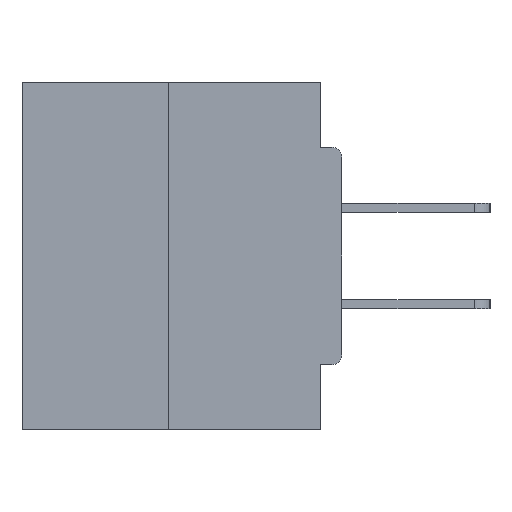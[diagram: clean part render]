
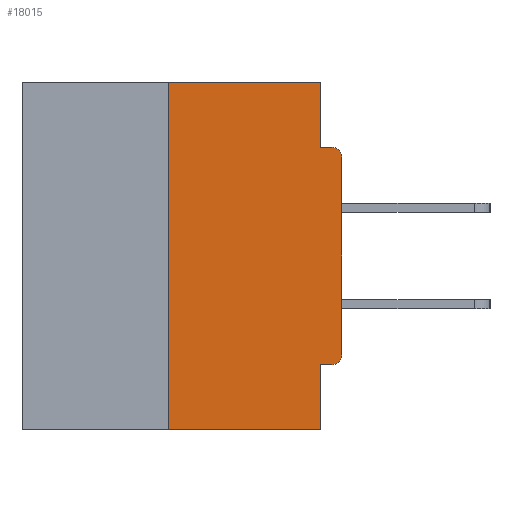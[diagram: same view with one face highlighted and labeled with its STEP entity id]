
A CAD part, left-side view. The second image highlights one B-rep face of the part: STEP entity #18015.
In plain terms, the highlighted planar face has unit normal (-1, 0, 0).
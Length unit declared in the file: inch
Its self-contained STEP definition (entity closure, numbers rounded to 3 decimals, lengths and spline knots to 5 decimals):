
#684 = VECTOR ( 'NONE', #2803, 39.37008 ) ;
#2041 = CARTESIAN_POINT ( 'NONE',  ( 0., 0., -0.1085 ) ) ;
#2444 = LINE ( 'NONE', #12914, #16984 ) ;
#2581 = DIRECTION ( 'NONE',  ( 0., 1., 0. ) ) ;
#2596 = VERTEX_POINT ( 'NONE', #25024 ) ;
#2803 = DIRECTION ( 'NONE',  ( 0., 0., -1. ) ) ;
#2924 = CARTESIAN_POINT ( 'NONE',  ( 0., 0.031, 0. ) ) ;
#6374 = CARTESIAN_POINT ( 'NONE',  ( 0., 0.015, -0.3915 ) ) ;
#7508 = ORIENTED_EDGE ( 'NONE', *, *, #24703, .F. ) ;
#7919 = VERTEX_POINT ( 'NONE', #28114 ) ;
#8001 = LINE ( 'NONE', #14122, #15034 ) ;
#8220 = CARTESIAN_POINT ( 'NONE',  ( 0., 0.46, 0. ) ) ;
#8406 = CIRCLE ( 'NONE', #10745, 0.015 ) ;
#8609 = DIRECTION ( 'NONE',  ( 0., -1., 0. ) ) ;
#8779 = CARTESIAN_POINT ( 'NONE',  ( 0., 0.031, -0.5 ) ) ;
#8786 = VERTEX_POINT ( 'NONE', #18698 ) ;
#9043 = VERTEX_POINT ( 'NONE', #23918 ) ;
#9921 = DIRECTION ( 'NONE',  ( 0., 0., -1. ) ) ;
#10245 = DIRECTION ( 'NONE',  ( 0., 0., 1. ) ) ;
#10745 = AXIS2_PLACEMENT_3D ( 'NONE', #6374, #18304, #21224 ) ;
#10990 = LINE ( 'NONE', #20159, #27864 ) ;
#11111 = DIRECTION ( 'NONE',  ( 1., 0., 0. ) ) ;
#11325 = VERTEX_POINT ( 'NONE', #27994 ) ;
#12914 = CARTESIAN_POINT ( 'NONE',  ( 0., 0., -0.0935 ) ) ;
#13152 = VERTEX_POINT ( 'NONE', #30198 ) ;
#13194 = DIRECTION ( 'NONE',  ( 0., 0., 1. ) ) ;
#13291 = LINE ( 'NONE', #37872, #15189 ) ;
#13634 = FACE_OUTER_BOUND ( 'NONE', #14030, .T. ) ;
#14030 = EDGE_LOOP ( 'NONE', ( #18086, #17177, #38280, #30702, #7508, #28239, #34104, #29452, #17872, #21770 ) ) ;
#14122 = CARTESIAN_POINT ( 'NONE',  ( 0., 0.25, 0. ) ) ;
#14210 = EDGE_CURVE ( 'NONE', #2596, #9043, #8406, .T. ) ;
#15034 = VECTOR ( 'NONE', #13194, 39.37008 ) ;
#15189 = VECTOR ( 'NONE', #20075, 39.37008 ) ;
#16087 = DIRECTION ( 'NONE',  ( 0., -1., 0. ) ) ;
#16645 = LINE ( 'NONE', #2924, #684 ) ;
#16984 = VECTOR ( 'NONE', #16087, 39.37008 ) ;
#17177 = ORIENTED_EDGE ( 'NONE', *, *, #32127, .F. ) ;
#17527 = VERTEX_POINT ( 'NONE', #18280 ) ;
#17872 = ORIENTED_EDGE ( 'NONE', *, *, #37528, .F. ) ;
#18015 = ADVANCED_FACE ( 'NONE', ( #13634 ), #34846, .F. ) ;
#18086 = ORIENTED_EDGE ( 'NONE', *, *, #26657, .F. ) ;
#18280 = CARTESIAN_POINT ( 'NONE',  ( 0., 0.031, -0.4065 ) ) ;
#18304 = DIRECTION ( 'NONE',  ( -1., 0., 0. ) ) ;
#18698 = CARTESIAN_POINT ( 'NONE',  ( 0., 0.031, 0. ) ) ;
#19701 = CARTESIAN_POINT ( 'NONE',  ( 0., 0.031, -0.5 ) ) ;
#20075 = DIRECTION ( 'NONE',  ( 0., -1., 0. ) ) ;
#20159 = CARTESIAN_POINT ( 'NONE',  ( 0., 0., -0.4065 ) ) ;
#21224 = DIRECTION ( 'NONE',  ( 0., 0., -1. ) ) ;
#21770 = ORIENTED_EDGE ( 'NONE', *, *, #29424, .F. ) ;
#21879 = CARTESIAN_POINT ( 'NONE',  ( 0., 0.015, -0.1085 ) ) ;
#22448 = VERTEX_POINT ( 'NONE', #35434 ) ;
#23524 = VECTOR ( 'NONE', #23744, 39.37008 ) ;
#23744 = DIRECTION ( 'NONE',  ( 0., 0., -1. ) ) ;
#23918 = CARTESIAN_POINT ( 'NONE',  ( 0., 0., -0.3915 ) ) ;
#24016 = VERTEX_POINT ( 'NONE', #2041 ) ;
#24703 = EDGE_CURVE ( 'NONE', #2596, #17527, #10990, .T. ) ;
#25024 = CARTESIAN_POINT ( 'NONE',  ( 0., 0.015, -0.4065 ) ) ;
#26657 = EDGE_CURVE ( 'NONE', #11325, #8786, #13291, .T. ) ;
#26974 = CARTESIAN_POINT ( 'NONE',  ( 0., 0.46, -0.5 ) ) ;
#27764 = DIRECTION ( 'NONE',  ( -1., 0., 0. ) ) ;
#27864 = VECTOR ( 'NONE', #2581, 39.37008 ) ;
#27994 = CARTESIAN_POINT ( 'NONE',  ( 0., 0.25, 0. ) ) ;
#28114 = CARTESIAN_POINT ( 'NONE',  ( 0., 0.031, -0.0935 ) ) ;
#28239 = ORIENTED_EDGE ( 'NONE', *, *, #14210, .T. ) ;
#28599 = CARTESIAN_POINT ( 'NONE',  ( 0., 0., 0. ) ) ;
#29424 = EDGE_CURVE ( 'NONE', #8786, #7919, #16645, .T. ) ;
#29452 = ORIENTED_EDGE ( 'NONE', *, *, #37098, .T. ) ;
#29627 = CIRCLE ( 'NONE', #30717, 0.015 ) ;
#30198 = CARTESIAN_POINT ( 'NONE',  ( 0., 0.25, -0.5 ) ) ;
#30702 = ORIENTED_EDGE ( 'NONE', *, *, #36808, .F. ) ;
#30717 = AXIS2_PLACEMENT_3D ( 'NONE', #21879, #27764, #9921 ) ;
#31597 = VERTEX_POINT ( 'NONE', #19701 ) ;
#31949 = LINE ( 'NONE', #8779, #23524 ) ;
#32127 = EDGE_CURVE ( 'NONE', #13152, #11325, #8001, .T. ) ;
#33195 = AXIS2_PLACEMENT_3D ( 'NONE', #8220, #11111, #37869 ) ;
#34104 = ORIENTED_EDGE ( 'NONE', *, *, #37985, .T. ) ;
#34175 = LINE ( 'NONE', #26974, #36525 ) ;
#34442 = EDGE_CURVE ( 'NONE', #13152, #31597, #34175, .T. ) ;
#34713 = LINE ( 'NONE', #28599, #37548 ) ;
#34846 = PLANE ( 'NONE',  #33195 ) ;
#35434 = CARTESIAN_POINT ( 'NONE',  ( 0., 0.015, -0.0935 ) ) ;
#36525 = VECTOR ( 'NONE', #8609, 39.37008 ) ;
#36808 = EDGE_CURVE ( 'NONE', #17527, #31597, #31949, .T. ) ;
#37098 = EDGE_CURVE ( 'NONE', #24016, #22448, #29627, .T. ) ;
#37528 = EDGE_CURVE ( 'NONE', #7919, #22448, #2444, .T. ) ;
#37548 = VECTOR ( 'NONE', #10245, 39.37008 ) ;
#37869 = DIRECTION ( 'NONE',  ( 0., 0., -1. ) ) ;
#37872 = CARTESIAN_POINT ( 'NONE',  ( 0., 0.46, 0. ) ) ;
#37985 = EDGE_CURVE ( 'NONE', #9043, #24016, #34713, .T. ) ;
#38280 = ORIENTED_EDGE ( 'NONE', *, *, #34442, .T. ) ;
